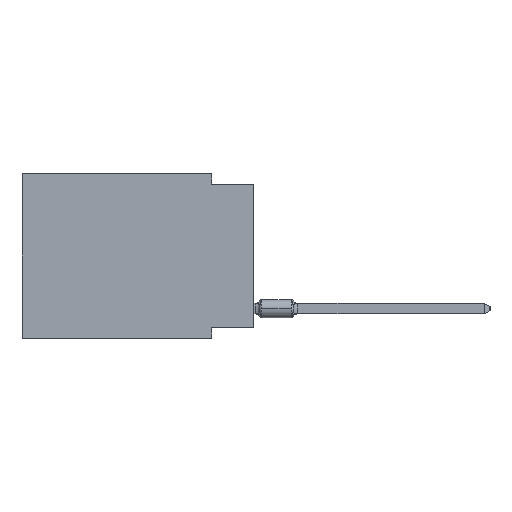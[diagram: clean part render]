
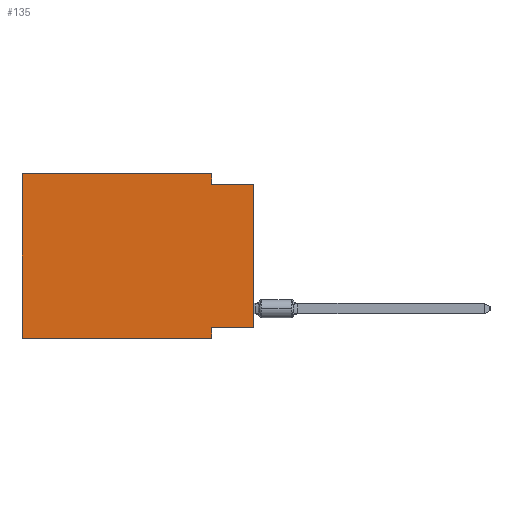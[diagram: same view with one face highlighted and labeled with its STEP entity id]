
A CAD part, left-side view. The second image highlights one B-rep face of the part: STEP entity #135.
In plain terms, the highlighted planar face has unit normal (-1, 0, 0).
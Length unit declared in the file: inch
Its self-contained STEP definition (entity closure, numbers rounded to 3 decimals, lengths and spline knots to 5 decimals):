
#13 = CARTESIAN_POINT ( 'NONE',  ( 0., 0.55, 0. ) ) ;
#135 = ADVANCED_FACE ( 'NONE', ( #6893 ), #9199, .F. ) ;
#378 = CARTESIAN_POINT ( 'NONE',  ( 0., 0.55, 0. ) ) ;
#757 = VERTEX_POINT ( 'NONE', #986 ) ;
#986 = CARTESIAN_POINT ( 'NONE',  ( 0., 0.1, -0.365 ) ) ;
#1097 = VECTOR ( 'NONE', #3554, 39.37008 ) ;
#1287 = EDGE_CURVE ( 'NONE', #5574, #8245, #3256, .T. ) ;
#1345 = ORIENTED_EDGE ( 'NONE', *, *, #1737, .F. ) ;
#1737 = EDGE_CURVE ( 'NONE', #1887, #5574, #9831, .T. ) ;
#1887 = VERTEX_POINT ( 'NONE', #12271 ) ;
#1975 = VERTEX_POINT ( 'NONE', #11627 ) ;
#2245 = EDGE_CURVE ( 'NONE', #3992, #757, #3489, .T. ) ;
#2336 = CARTESIAN_POINT ( 'NONE',  ( 0., 0.1, 0. ) ) ;
#2343 = EDGE_CURVE ( 'NONE', #757, #8585, #2705, .T. ) ;
#2435 = DIRECTION ( 'NONE',  ( 0., -1., 0. ) ) ;
#2478 = ORIENTED_EDGE ( 'NONE', *, *, #3636, .T. ) ;
#2533 = DIRECTION ( 'NONE',  ( 0., 0., -1. ) ) ;
#2705 = LINE ( 'NONE', #9564, #11876 ) ;
#3068 = ORIENTED_EDGE ( 'NONE', *, *, #2245, .F. ) ;
#3256 = LINE ( 'NONE', #3320, #11840 ) ;
#3320 = CARTESIAN_POINT ( 'NONE',  ( 0., 0.1, 0. ) ) ;
#3367 = DIRECTION ( 'NONE',  ( 0., -1., 0. ) ) ;
#3489 = LINE ( 'NONE', #9013, #1097 ) ;
#3554 = DIRECTION ( 'NONE',  ( 0., 1., 0. ) ) ;
#3558 = EDGE_LOOP ( 'NONE', ( #11781, #14109, #3911, #1345, #7048, #2478, #6569, #3068 ) ) ;
#3636 = EDGE_CURVE ( 'NONE', #8976, #8585, #7957, .T. ) ;
#3911 = ORIENTED_EDGE ( 'NONE', *, *, #1287, .F. ) ;
#3992 = VERTEX_POINT ( 'NONE', #13439 ) ;
#4155 = CARTESIAN_POINT ( 'NONE',  ( 0., 0.1, -0.39 ) ) ;
#4431 = DIRECTION ( 'NONE',  ( 0., 0., 1. ) ) ;
#4978 = LINE ( 'NONE', #10451, #9090 ) ;
#5269 = VECTOR ( 'NONE', #11614, 39.37008 ) ;
#5547 = DIRECTION ( 'NONE',  ( 0., 0., -1. ) ) ;
#5574 = VERTEX_POINT ( 'NONE', #2336 ) ;
#6341 = DIRECTION ( 'NONE',  ( 0., 0., -1. ) ) ;
#6569 = ORIENTED_EDGE ( 'NONE', *, *, #2343, .F. ) ;
#6893 = FACE_OUTER_BOUND ( 'NONE', #3558, .T. ) ;
#7048 = ORIENTED_EDGE ( 'NONE', *, *, #7697, .F. ) ;
#7697 = EDGE_CURVE ( 'NONE', #8976, #1887, #4978, .T. ) ;
#7957 = LINE ( 'NONE', #11061, #11584 ) ;
#8245 = VERTEX_POINT ( 'NONE', #14137 ) ;
#8582 = AXIS2_PLACEMENT_3D ( 'NONE', #378, #12214, #2533 ) ;
#8585 = VERTEX_POINT ( 'NONE', #4155 ) ;
#8806 = EDGE_CURVE ( 'NONE', #3992, #1975, #8869, .T. ) ;
#8869 = LINE ( 'NONE', #10972, #13236 ) ;
#8976 = VERTEX_POINT ( 'NONE', #11262 ) ;
#9013 = CARTESIAN_POINT ( 'NONE',  ( 0., 0., -0.365 ) ) ;
#9090 = VECTOR ( 'NONE', #13735, 39.37008 ) ;
#9199 = PLANE ( 'NONE',  #8582 ) ;
#9564 = CARTESIAN_POINT ( 'NONE',  ( 0., 0.1, -0.39 ) ) ;
#9796 = VECTOR ( 'NONE', #3367, 39.37008 ) ;
#9831 = LINE ( 'NONE', #13, #9796 ) ;
#10451 = CARTESIAN_POINT ( 'NONE',  ( 0., 0.55, 0. ) ) ;
#10928 = EDGE_CURVE ( 'NONE', #8245, #1975, #13488, .T. ) ;
#10972 = CARTESIAN_POINT ( 'NONE',  ( 0., 0., 0. ) ) ;
#11061 = CARTESIAN_POINT ( 'NONE',  ( 0., 0.55, -0.39 ) ) ;
#11262 = CARTESIAN_POINT ( 'NONE',  ( 0., 0.55, -0.39 ) ) ;
#11584 = VECTOR ( 'NONE', #2435, 39.37008 ) ;
#11614 = DIRECTION ( 'NONE',  ( 0., -1., 0. ) ) ;
#11627 = CARTESIAN_POINT ( 'NONE',  ( 0., 0., -0.025 ) ) ;
#11781 = ORIENTED_EDGE ( 'NONE', *, *, #8806, .T. ) ;
#11840 = VECTOR ( 'NONE', #5547, 39.37008 ) ;
#11876 = VECTOR ( 'NONE', #6341, 39.37008 ) ;
#12214 = DIRECTION ( 'NONE',  ( 1., 0., 0. ) ) ;
#12271 = CARTESIAN_POINT ( 'NONE',  ( 0., 0.55, 0. ) ) ;
#12899 = CARTESIAN_POINT ( 'NONE',  ( 0., 0., -0.025 ) ) ;
#13236 = VECTOR ( 'NONE', #4431, 39.37008 ) ;
#13439 = CARTESIAN_POINT ( 'NONE',  ( 0., 0., -0.365 ) ) ;
#13488 = LINE ( 'NONE', #12899, #5269 ) ;
#13735 = DIRECTION ( 'NONE',  ( 0., 0., 1. ) ) ;
#14109 = ORIENTED_EDGE ( 'NONE', *, *, #10928, .F. ) ;
#14137 = CARTESIAN_POINT ( 'NONE',  ( 0., 0.1, -0.025 ) ) ;
